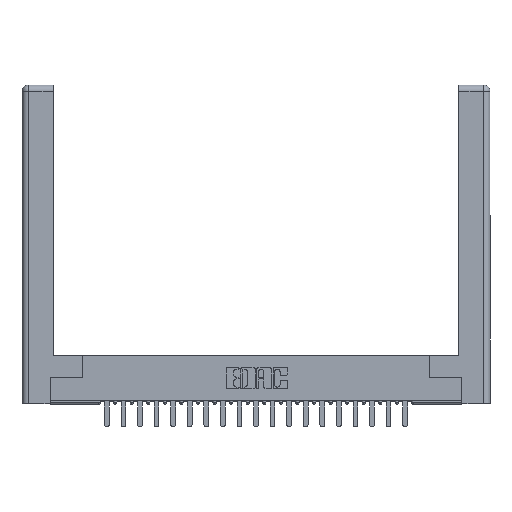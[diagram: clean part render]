
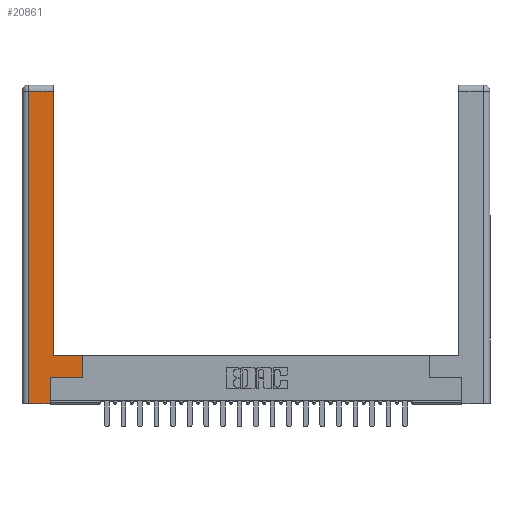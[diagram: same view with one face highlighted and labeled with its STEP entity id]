
A CAD part, top view. The second image highlights one B-rep face of the part: STEP entity #20861.
In plain terms, the highlighted planar face has unit normal (0, 0, 1).
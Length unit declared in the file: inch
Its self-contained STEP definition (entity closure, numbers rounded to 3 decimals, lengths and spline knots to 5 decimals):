
#798 = DIRECTION ( 'NONE',  ( -1., 0., 0. ) ) ;
#1113 = EDGE_CURVE ( 'NONE', #10271, #16333, #19714, .T. ) ;
#1337 = ORIENTED_EDGE ( 'NONE', *, *, #1113, .T. ) ;
#1839 = CARTESIAN_POINT ( 'NONE',  ( 0.565, 0.45, 0. ) ) ;
#1874 = EDGE_CURVE ( 'NONE', #18995, #7031, #8726, .T. ) ;
#1971 = EDGE_CURVE ( 'NONE', #16333, #18995, #23402, .T. ) ;
#2595 = DIRECTION ( 'NONE',  ( 0., 1., 0. ) ) ;
#2869 = EDGE_CURVE ( 'NONE', #17950, #25573, #7119, .T. ) ;
#3661 = LINE ( 'NONE', #24848, #24335 ) ;
#4000 = DIRECTION ( 'NONE',  ( 1., 0., 0. ) ) ;
#4047 = LINE ( 'NONE', #15305, #5317 ) ;
#4859 = EDGE_CURVE ( 'NONE', #6518, #10271, #17647, .T. ) ;
#5179 = CARTESIAN_POINT ( 'NONE',  ( 0.265, 0.245, 0. ) ) ;
#5317 = VECTOR ( 'NONE', #25332, 39.37008 ) ;
#6093 = VECTOR ( 'NONE', #2595, 39.37008 ) ;
#6518 = VERTEX_POINT ( 'NONE', #21306 ) ;
#6561 = VECTOR ( 'NONE', #13449, 39.37008 ) ;
#7031 = VERTEX_POINT ( 'NONE', #23388 ) ;
#7119 = LINE ( 'NONE', #17437, #8356 ) ;
#7162 = VECTOR ( 'NONE', #19696, 39.37008 ) ;
#8215 = ORIENTED_EDGE ( 'NONE', *, *, #9410, .T. ) ;
#8348 = AXIS2_PLACEMENT_3D ( 'NONE', #16644, #16475, #798 ) ;
#8356 = VECTOR ( 'NONE', #17344, 39.37008 ) ;
#8397 = CARTESIAN_POINT ( 'NONE',  ( 0.265, 0.245, 0. ) ) ;
#8726 = LINE ( 'NONE', #13529, #6561 ) ;
#9410 = EDGE_CURVE ( 'NONE', #17908, #6518, #3661, .T. ) ;
#10197 = VECTOR ( 'NONE', #21057, 39.37008 ) ;
#10271 = VERTEX_POINT ( 'NONE', #5179 ) ;
#10812 = LINE ( 'NONE', #15182, #10197 ) ;
#10953 = EDGE_CURVE ( 'NONE', #25573, #17908, #10812, .T. ) ;
#12269 = ORIENTED_EDGE ( 'NONE', *, *, #10953, .T. ) ;
#13182 = CARTESIAN_POINT ( 'NONE',  ( 0.0615, 2.94, 0. ) ) ;
#13449 = DIRECTION ( 'NONE',  ( -1., 0., 0. ) ) ;
#13529 = CARTESIAN_POINT ( 'NONE',  ( 0.295, 0.45, 0. ) ) ;
#14032 = CARTESIAN_POINT ( 'NONE',  ( 0.0615, 0., 0. ) ) ;
#14898 = DIRECTION ( 'NONE',  ( 1., 0., 0. ) ) ;
#15182 = CARTESIAN_POINT ( 'NONE',  ( 0.0615, 0., 0. ) ) ;
#15305 = CARTESIAN_POINT ( 'NONE',  ( 0.295, 3., 0. ) ) ;
#16264 = CARTESIAN_POINT ( 'NONE',  ( 0.295, 2.94, 0. ) ) ;
#16333 = VERTEX_POINT ( 'NONE', #18659 ) ;
#16475 = DIRECTION ( 'NONE',  ( 0., 0., -1. ) ) ;
#16644 = CARTESIAN_POINT ( 'NONE',  ( 0., 0., 0. ) ) ;
#16728 = PLANE ( 'NONE',  #8348 ) ;
#17344 = DIRECTION ( 'NONE',  ( -1., 0., 0. ) ) ;
#17437 = CARTESIAN_POINT ( 'NONE',  ( 0.0615, 2.94, 0. ) ) ;
#17647 = LINE ( 'NONE', #8397, #6093 ) ;
#17908 = VERTEX_POINT ( 'NONE', #14032 ) ;
#17950 = VERTEX_POINT ( 'NONE', #16264 ) ;
#18569 = CARTESIAN_POINT ( 'NONE',  ( 0.565, 0.45, 0. ) ) ;
#18659 = CARTESIAN_POINT ( 'NONE',  ( 0.565, 0.245, 0. ) ) ;
#18995 = VERTEX_POINT ( 'NONE', #18569 ) ;
#19465 = ORIENTED_EDGE ( 'NONE', *, *, #1874, .T. ) ;
#19696 = DIRECTION ( 'NONE',  ( 0., 1., 0. ) ) ;
#19714 = LINE ( 'NONE', #20296, #24672 ) ;
#19833 = EDGE_CURVE ( 'NONE', #7031, #17950, #4047, .T. ) ;
#20296 = CARTESIAN_POINT ( 'NONE',  ( 0.565, 0.245, 0. ) ) ;
#20861 = ADVANCED_FACE ( 'NONE', ( #21255 ), #16728, .F. ) ;
#20864 = ORIENTED_EDGE ( 'NONE', *, *, #4859, .T. ) ;
#21057 = DIRECTION ( 'NONE',  ( 0., -1., 0. ) ) ;
#21255 = FACE_OUTER_BOUND ( 'NONE', #21712, .T. ) ;
#21306 = CARTESIAN_POINT ( 'NONE',  ( 0.265, 0., 0. ) ) ;
#21712 = EDGE_LOOP ( 'NONE', ( #24516, #21881, #12269, #8215, #20864, #1337, #25254, #19465 ) ) ;
#21881 = ORIENTED_EDGE ( 'NONE', *, *, #2869, .T. ) ;
#23388 = CARTESIAN_POINT ( 'NONE',  ( 0.295, 0.45, 0. ) ) ;
#23402 = LINE ( 'NONE', #1839, #7162 ) ;
#24335 = VECTOR ( 'NONE', #14898, 39.37008 ) ;
#24516 = ORIENTED_EDGE ( 'NONE', *, *, #19833, .T. ) ;
#24672 = VECTOR ( 'NONE', #4000, 39.37008 ) ;
#24848 = CARTESIAN_POINT ( 'NONE',  ( 0.265, 0., 0. ) ) ;
#25254 = ORIENTED_EDGE ( 'NONE', *, *, #1971, .T. ) ;
#25332 = DIRECTION ( 'NONE',  ( 0., 1., 0. ) ) ;
#25573 = VERTEX_POINT ( 'NONE', #13182 ) ;
